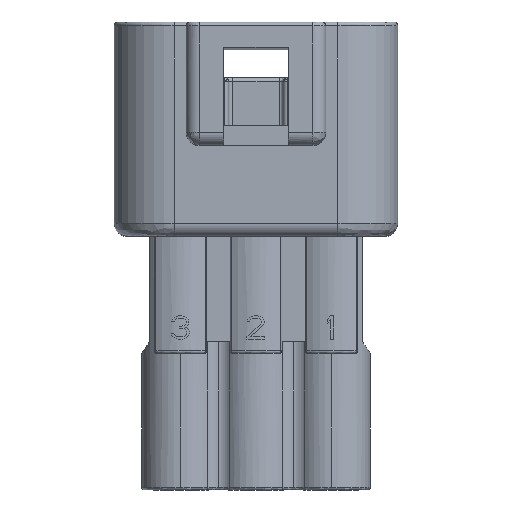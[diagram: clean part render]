
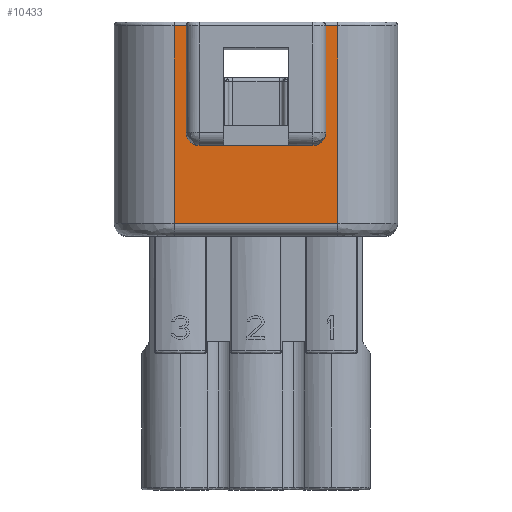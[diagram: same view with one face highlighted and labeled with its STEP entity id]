
A CAD part, front view. The second image highlights one B-rep face of the part: STEP entity #10433.
In plain terms, the highlighted planar face has unit normal (0, -1, 0).
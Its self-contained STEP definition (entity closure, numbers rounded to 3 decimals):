
#99 = CARTESIAN_POINT ( 'NONE',  ( 4.375, -6.3, -9.5 ) ) ;
#271 = ORIENTED_EDGE ( 'NONE', *, *, #16981, .T. ) ;
#361 = ORIENTED_EDGE ( 'NONE', *, *, #18586, .T. ) ;
#410 = VECTOR ( 'NONE', #3051, 1000. ) ;
#448 = CARTESIAN_POINT ( 'NONE',  ( 10.9, -6.3, -0.3 ) ) ;
#713 = EDGE_CURVE ( 'NONE', #5762, #1022, #5730, .T. ) ;
#923 = DIRECTION ( 'NONE',  ( 0., 0., -1. ) ) ;
#1022 = VERTEX_POINT ( 'NONE', #2648 ) ;
#1155 = VERTEX_POINT ( 'NONE', #19557 ) ;
#1350 = DIRECTION ( 'NONE',  ( -1., 0., 0. ) ) ;
#1450 = ORIENTED_EDGE ( 'NONE', *, *, #5084, .T. ) ;
#1497 = EDGE_CURVE ( 'NONE', #1022, #16469, #10668, .T. ) ;
#1759 = EDGE_CURVE ( 'NONE', #1155, #18830, #14916, .T. ) ;
#1779 = VECTOR ( 'NONE', #10204, 1000. ) ;
#1991 = CARTESIAN_POINT ( 'NONE',  ( -6.3, -6.3, -38.009 ) ) ;
#2093 = DIRECTION ( 'NONE',  ( 0., 0., 1. ) ) ;
#2249 = CARTESIAN_POINT ( 'NONE',  ( -4.375, -6.3, -8.5 ) ) ;
#2648 = CARTESIAN_POINT ( 'NONE',  ( 5.375, -6.3, -0.3 ) ) ;
#3051 = DIRECTION ( 'NONE',  ( -1., 0., 0. ) ) ;
#3438 = DIRECTION ( 'NONE',  ( -1., 0., 0. ) ) ;
#3797 = CARTESIAN_POINT ( 'NONE',  ( 6.3, -6.3, 0. ) ) ;
#4026 = DIRECTION ( 'NONE',  ( -1., 0., 0. ) ) ;
#4067 = CARTESIAN_POINT ( 'NONE',  ( 10.9, -6.3, -0.3 ) ) ;
#4190 = EDGE_CURVE ( 'NONE', #7558, #13181, #19500, .T. ) ;
#4557 = VECTOR ( 'NONE', #18105, 1000. ) ;
#4575 = CARTESIAN_POINT ( 'NONE',  ( 6.349, -6.3, -15.5 ) ) ;
#4734 = VERTEX_POINT ( 'NONE', #18631 ) ;
#4921 = CARTESIAN_POINT ( 'NONE',  ( 6.3, -6.3, -15.5 ) ) ;
#4938 = EDGE_CURVE ( 'NONE', #8526, #5762, #18682, .T. ) ;
#4943 = EDGE_CURVE ( 'NONE', #4734, #1155, #18471, .T. ) ;
#5084 = EDGE_CURVE ( 'NONE', #16469, #13682, #7210, .T. ) ;
#5730 = LINE ( 'NONE', #4067, #1779 ) ;
#5762 = VERTEX_POINT ( 'NONE', #15329 ) ;
#6034 = CARTESIAN_POINT ( 'NONE',  ( 4.375, -6.3, -8.5 ) ) ;
#6533 = ORIENTED_EDGE ( 'NONE', *, *, #4938, .T. ) ;
#7136 = FACE_OUTER_BOUND ( 'NONE', #10272, .T. ) ;
#7210 = CIRCLE ( 'NONE', #19137, 1. ) ;
#7558 = VERTEX_POINT ( 'NONE', #19135 ) ;
#8229 = ORIENTED_EDGE ( 'NONE', *, *, #4943, .T. ) ;
#8526 = VERTEX_POINT ( 'NONE', #4921 ) ;
#8777 = DIRECTION ( 'NONE',  ( 0., 1., 0. ) ) ;
#8910 = CARTESIAN_POINT ( 'NONE',  ( 5.375, -6.3, 0. ) ) ;
#9259 = DIRECTION ( 'NONE',  ( 1., 0., 0. ) ) ;
#9444 = LINE ( 'NONE', #4575, #18786 ) ;
#9719 = ORIENTED_EDGE ( 'NONE', *, *, #1759, .T. ) ;
#9902 = ORIENTED_EDGE ( 'NONE', *, *, #713, .T. ) ;
#10161 = PLANE ( 'NONE',  #14121 ) ;
#10204 = DIRECTION ( 'NONE',  ( -1., 0., 0. ) ) ;
#10272 = EDGE_LOOP ( 'NONE', ( #9719, #361, #12552, #11832, #6533, #9902, #15992, #1450, #271, #8229 ) ) ;
#10433 = ADVANCED_FACE ( 'NONE', ( #7136 ), #10161, .T. ) ;
#10668 = LINE ( 'NONE', #8910, #14296 ) ;
#10877 = VECTOR ( 'NONE', #17814, 1000. ) ;
#10947 = LINE ( 'NONE', #12906, #410 ) ;
#11706 = CARTESIAN_POINT ( 'NONE',  ( -5.375, -6.3, 0. ) ) ;
#11832 = ORIENTED_EDGE ( 'NONE', *, *, #12228, .F. ) ;
#12228 = EDGE_CURVE ( 'NONE', #8526, #7558, #9444, .T. ) ;
#12552 = ORIENTED_EDGE ( 'NONE', *, *, #4190, .F. ) ;
#12906 = CARTESIAN_POINT ( 'NONE',  ( 10.9, -6.3, -9.5 ) ) ;
#13181 = VERTEX_POINT ( 'NONE', #17141 ) ;
#13470 = CARTESIAN_POINT ( 'NONE',  ( 10.9, -6.3, 0. ) ) ;
#13682 = VERTEX_POINT ( 'NONE', #99 ) ;
#13804 = VECTOR ( 'NONE', #2093, 1000. ) ;
#14121 = AXIS2_PLACEMENT_3D ( 'NONE', #13470, #19777, #4026 ) ;
#14296 = VECTOR ( 'NONE', #923, 1000. ) ;
#14639 = VECTOR ( 'NONE', #16222, 1000. ) ;
#14765 = LINE ( 'NONE', #448, #14639 ) ;
#14916 = LINE ( 'NONE', #11706, #10877 ) ;
#15329 = CARTESIAN_POINT ( 'NONE',  ( 6.3, -6.3, -0.3 ) ) ;
#15992 = ORIENTED_EDGE ( 'NONE', *, *, #1497, .T. ) ;
#16222 = DIRECTION ( 'NONE',  ( -1., 0., 0. ) ) ;
#16469 = VERTEX_POINT ( 'NONE', #18401 ) ;
#16981 = EDGE_CURVE ( 'NONE', #13682, #4734, #10947, .T. ) ;
#17141 = CARTESIAN_POINT ( 'NONE',  ( -6.3, -6.3, -0.3 ) ) ;
#17227 = CARTESIAN_POINT ( 'NONE',  ( -5.375, -6.3, -0.3 ) ) ;
#17238 = DIRECTION ( 'NONE',  ( 0., 1., 0. ) ) ;
#17814 = DIRECTION ( 'NONE',  ( 0., 0., 1. ) ) ;
#18105 = DIRECTION ( 'NONE',  ( 0., 0., 1. ) ) ;
#18125 = AXIS2_PLACEMENT_3D ( 'NONE', #2249, #8777, #9259 ) ;
#18401 = CARTESIAN_POINT ( 'NONE',  ( 5.375, -6.3, -8.5 ) ) ;
#18471 = CIRCLE ( 'NONE', #18125, 1. ) ;
#18586 = EDGE_CURVE ( 'NONE', #18830, #13181, #14765, .T. ) ;
#18631 = CARTESIAN_POINT ( 'NONE',  ( -4.375, -6.3, -9.5 ) ) ;
#18682 = LINE ( 'NONE', #3797, #4557 ) ;
#18786 = VECTOR ( 'NONE', #1350, 1000. ) ;
#18830 = VERTEX_POINT ( 'NONE', #17227 ) ;
#19135 = CARTESIAN_POINT ( 'NONE',  ( -6.3, -6.3, -15.5 ) ) ;
#19137 = AXIS2_PLACEMENT_3D ( 'NONE', #6034, #17238, #3438 ) ;
#19500 = LINE ( 'NONE', #1991, #13804 ) ;
#19557 = CARTESIAN_POINT ( 'NONE',  ( -5.375, -6.3, -8.5 ) ) ;
#19777 = DIRECTION ( 'NONE',  ( 0., -1., 0. ) ) ;
